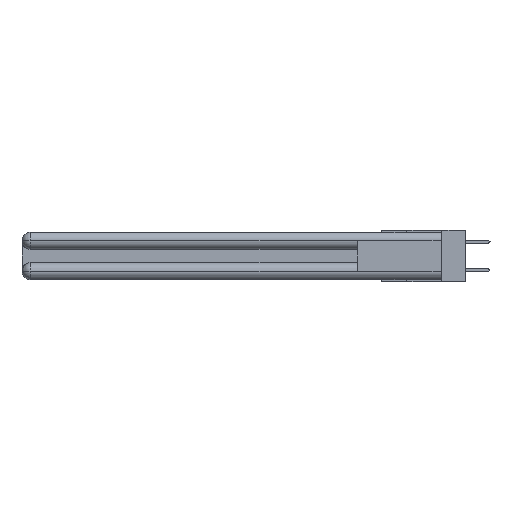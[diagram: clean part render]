
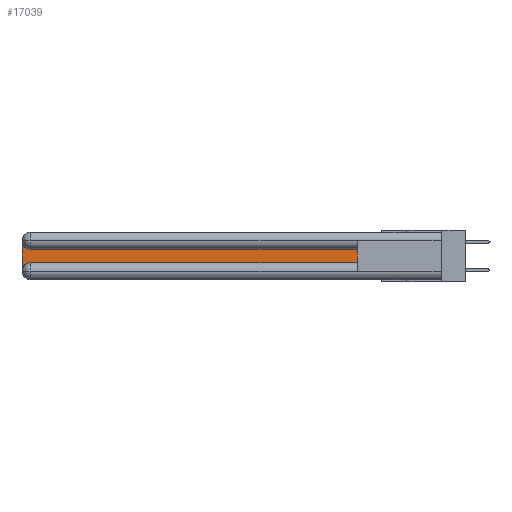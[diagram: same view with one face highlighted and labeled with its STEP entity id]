
A CAD part, left-side view. The second image highlights one B-rep face of the part: STEP entity #17039.
In plain terms, the highlighted planar face has unit normal (-1, 0, 0).
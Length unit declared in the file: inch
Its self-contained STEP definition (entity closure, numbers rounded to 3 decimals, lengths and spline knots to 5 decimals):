
#445 = EDGE_CURVE ( 'NONE', #21549, #33891, #22914, .T. ) ;
#1121 = DIRECTION ( 'NONE',  ( 0., 0., 1. ) ) ;
#1439 = ORIENTED_EDGE ( 'NONE', *, *, #34474, .T. ) ;
#1483 = CARTESIAN_POINT ( 'NONE',  ( 0.075, 3., -0.1225 ) ) ;
#1535 = AXIS2_PLACEMENT_3D ( 'NONE', #25287, #9020, #6380 ) ;
#1732 = EDGE_LOOP ( 'NONE', ( #1439, #29334, #22613, #19567, #6519, #16144 ) ) ;
#1776 = CARTESIAN_POINT ( 'NONE',  ( 0.075, 2.94, -0.0625 ) ) ;
#1890 = VECTOR ( 'NONE', #12740, 39.37008 ) ;
#2225 = EDGE_CURVE ( 'NONE', #24855, #34703, #15921, .T. ) ;
#4380 = EDGE_CURVE ( 'NONE', #5113, #21549, #26290, .T. ) ;
#5113 = VERTEX_POINT ( 'NONE', #27527 ) ;
#5169 = AXIS2_PLACEMENT_3D ( 'NONE', #1776, #10034, #20818 ) ;
#6380 = DIRECTION ( 'NONE',  ( 0., 0., -1. ) ) ;
#6519 = ORIENTED_EDGE ( 'NONE', *, *, #4380, .T. ) ;
#6672 = EDGE_CURVE ( 'NONE', #27855, #24855, #14512, .T. ) ;
#9020 = DIRECTION ( 'NONE',  ( 1., 0., 0. ) ) ;
#9735 = DIRECTION ( 'NONE',  ( 0., 0., -1. ) ) ;
#9870 = CARTESIAN_POINT ( 'NONE',  ( 0.075, 3., -0.2775 ) ) ;
#10034 = DIRECTION ( 'NONE',  ( 1., 0., 0. ) ) ;
#11772 = CARTESIAN_POINT ( 'NONE',  ( 0.075, 0.6, -0.1225 ) ) ;
#12740 = DIRECTION ( 'NONE',  ( 0., -1., 0. ) ) ;
#13528 = FACE_OUTER_BOUND ( 'NONE', #1732, .T. ) ;
#14512 = CIRCLE ( 'NONE', #5169, 0.06 ) ;
#14527 = AXIS2_PLACEMENT_3D ( 'NONE', #1483, #15231, #9735 ) ;
#15231 = DIRECTION ( 'NONE',  ( 1., 0., 0. ) ) ;
#15921 = LINE ( 'NONE', #23348, #19755 ) ;
#16144 = ORIENTED_EDGE ( 'NONE', *, *, #445, .T. ) ;
#16740 = CARTESIAN_POINT ( 'NONE',  ( 0.075, 0.6, -0.2175 ) ) ;
#16884 = LINE ( 'NONE', #11772, #25851 ) ;
#17039 = ADVANCED_FACE ( 'NONE', ( #13528 ), #34237, .F. ) ;
#17426 = CARTESIAN_POINT ( 'NONE',  ( 0.075, 3., -0.0625 ) ) ;
#19567 = ORIENTED_EDGE ( 'NONE', *, *, #21163, .T. ) ;
#19755 = VECTOR ( 'NONE', #23592, 39.37008 ) ;
#20818 = DIRECTION ( 'NONE',  ( 0., 0., -1. ) ) ;
#21163 = EDGE_CURVE ( 'NONE', #34703, #5113, #30394, .T. ) ;
#21549 = VERTEX_POINT ( 'NONE', #16740 ) ;
#22613 = ORIENTED_EDGE ( 'NONE', *, *, #2225, .T. ) ;
#22914 = LINE ( 'NONE', #30304, #24167 ) ;
#23348 = CARTESIAN_POINT ( 'NONE',  ( 0.075, 3., -0.2175 ) ) ;
#23592 = DIRECTION ( 'NONE',  ( 0., 0., -1. ) ) ;
#24167 = VECTOR ( 'NONE', #1121, 39.37008 ) ;
#24855 = VERTEX_POINT ( 'NONE', #17426 ) ;
#25287 = CARTESIAN_POINT ( 'NONE',  ( 0.075, 2.94, -0.2775 ) ) ;
#25851 = VECTOR ( 'NONE', #28626, 39.37008 ) ;
#26273 = CARTESIAN_POINT ( 'NONE',  ( 0.075, 0.6, -0.2175 ) ) ;
#26290 = LINE ( 'NONE', #26273, #1890 ) ;
#27527 = CARTESIAN_POINT ( 'NONE',  ( 0.075, 2.94, -0.2175 ) ) ;
#27855 = VERTEX_POINT ( 'NONE', #30735 ) ;
#28626 = DIRECTION ( 'NONE',  ( 0., 1., 0. ) ) ;
#29334 = ORIENTED_EDGE ( 'NONE', *, *, #6672, .T. ) ;
#30304 = CARTESIAN_POINT ( 'NONE',  ( 0.075, 0.6, -0.2175 ) ) ;
#30394 = CIRCLE ( 'NONE', #1535, 0.06 ) ;
#30735 = CARTESIAN_POINT ( 'NONE',  ( 0.075, 2.94, -0.1225 ) ) ;
#32021 = CARTESIAN_POINT ( 'NONE',  ( 0.075, 0.6, -0.1225 ) ) ;
#33891 = VERTEX_POINT ( 'NONE', #32021 ) ;
#34237 = PLANE ( 'NONE',  #14527 ) ;
#34474 = EDGE_CURVE ( 'NONE', #33891, #27855, #16884, .T. ) ;
#34703 = VERTEX_POINT ( 'NONE', #9870 ) ;
